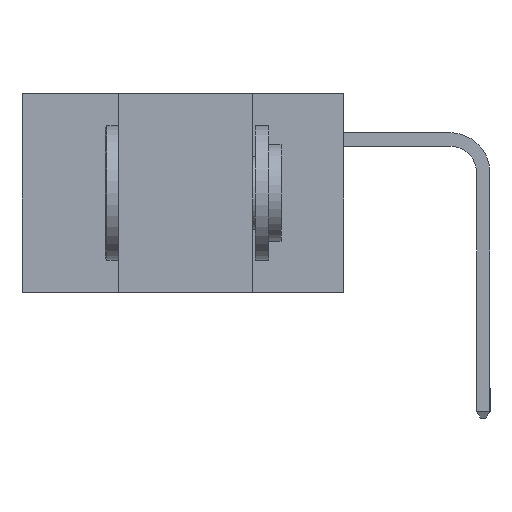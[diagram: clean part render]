
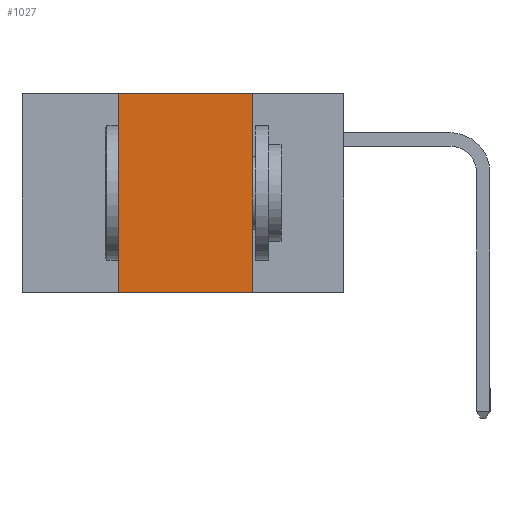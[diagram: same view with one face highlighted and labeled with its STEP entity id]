
A CAD part, left-side view. The second image highlights one B-rep face of the part: STEP entity #1027.
In plain terms, the highlighted planar face has unit normal (-1, 0, 0).
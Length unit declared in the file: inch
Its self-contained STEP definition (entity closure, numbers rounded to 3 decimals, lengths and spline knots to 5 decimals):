
#1027 = ADVANCED_FACE ( 'NONE', ( #2651 ), #18221, .F. ) ;
#1409 = CARTESIAN_POINT ( 'NONE',  ( 0., 0.42, -0.37 ) ) ;
#1416 = VECTOR ( 'NONE', #16783, 39.37008 ) ;
#1469 = CARTESIAN_POINT ( 'NONE',  ( 0., 0.17, 0. ) ) ;
#1728 = VERTEX_POINT ( 'NONE', #1409 ) ;
#2327 = EDGE_CURVE ( 'NONE', #13439, #6316, #10666, .T. ) ;
#2501 = VERTEX_POINT ( 'NONE', #15234 ) ;
#2651 = FACE_OUTER_BOUND ( 'NONE', #13767, .T. ) ;
#3978 = VECTOR ( 'NONE', #17804, 39.37008 ) ;
#4549 = LINE ( 'NONE', #23152, #3978 ) ;
#5803 = DIRECTION ( 'NONE',  ( 1., 0., 0. ) ) ;
#5824 = ORIENTED_EDGE ( 'NONE', *, *, #21547, .T. ) ;
#6316 = VERTEX_POINT ( 'NONE', #16425 ) ;
#6557 = EDGE_CURVE ( 'NONE', #1728, #13439, #15140, .T. ) ;
#10021 = LINE ( 'NONE', #1469, #19616 ) ;
#10666 = LINE ( 'NONE', #13733, #1416 ) ;
#11504 = EDGE_CURVE ( 'NONE', #6316, #2501, #10021, .T. ) ;
#13115 = CARTESIAN_POINT ( 'NONE',  ( 0., 0.42, 0. ) ) ;
#13157 = DIRECTION ( 'NONE',  ( 0., 0., 1. ) ) ;
#13439 = VERTEX_POINT ( 'NONE', #20132 ) ;
#13733 = CARTESIAN_POINT ( 'NONE',  ( 0., 0.6, 0. ) ) ;
#13767 = EDGE_LOOP ( 'NONE', ( #18603, #14429, #19162, #5824 ) ) ;
#14346 = DIRECTION ( 'NONE',  ( 0., 0., -1. ) ) ;
#14429 = ORIENTED_EDGE ( 'NONE', *, *, #2327, .F. ) ;
#14583 = VECTOR ( 'NONE', #13157, 39.37008 ) ;
#15140 = LINE ( 'NONE', #13115, #14583 ) ;
#15234 = CARTESIAN_POINT ( 'NONE',  ( 0., 0.17, -0.37 ) ) ;
#16425 = CARTESIAN_POINT ( 'NONE',  ( 0., 0.17, 0. ) ) ;
#16783 = DIRECTION ( 'NONE',  ( 0., -1., 0. ) ) ;
#17246 = CARTESIAN_POINT ( 'NONE',  ( 0., 0.6, 0. ) ) ;
#17804 = DIRECTION ( 'NONE',  ( 0., -1., 0. ) ) ;
#18221 = PLANE ( 'NONE',  #21317 ) ;
#18603 = ORIENTED_EDGE ( 'NONE', *, *, #11504, .F. ) ;
#19162 = ORIENTED_EDGE ( 'NONE', *, *, #6557, .F. ) ;
#19616 = VECTOR ( 'NONE', #14346, 39.37008 ) ;
#19990 = DIRECTION ( 'NONE',  ( 0., 0., -1. ) ) ;
#20132 = CARTESIAN_POINT ( 'NONE',  ( 0., 0.42, 0. ) ) ;
#21317 = AXIS2_PLACEMENT_3D ( 'NONE', #17246, #5803, #19990 ) ;
#21547 = EDGE_CURVE ( 'NONE', #1728, #2501, #4549, .T. ) ;
#23152 = CARTESIAN_POINT ( 'NONE',  ( 0., 0.6, -0.37 ) ) ;
